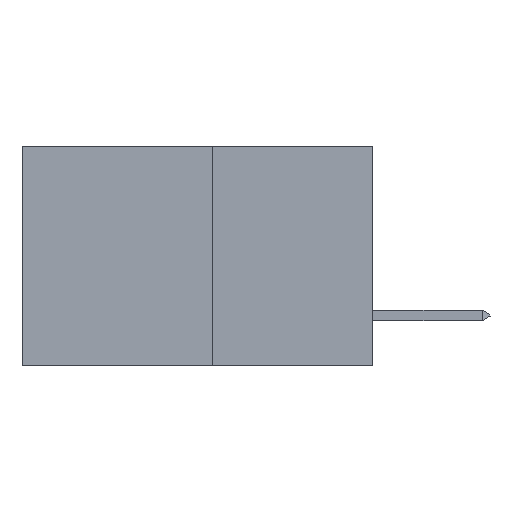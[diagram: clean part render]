
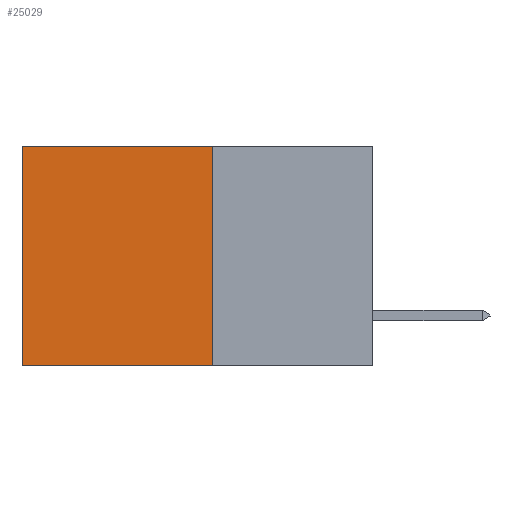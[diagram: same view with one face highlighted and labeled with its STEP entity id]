
A CAD part, left-side view. The second image highlights one B-rep face of the part: STEP entity #25029.
In plain terms, the highlighted planar face has unit normal (-1, 0, 0).
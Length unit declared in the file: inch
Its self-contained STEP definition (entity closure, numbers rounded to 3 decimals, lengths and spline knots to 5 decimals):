
#195 = LINE ( 'NONE', #1239, #15987 ) ;
#360 = LINE ( 'NONE', #1048, #6505 ) ;
#1048 = CARTESIAN_POINT ( 'NONE',  ( 0.277, 0.27, -0.37 ) ) ;
#1239 = CARTESIAN_POINT ( 'NONE',  ( 0.277, 0.27, 0. ) ) ;
#3177 = VERTEX_POINT ( 'NONE', #15548 ) ;
#3860 = CARTESIAN_POINT ( 'NONE',  ( 0.277, 0.27, -0.37 ) ) ;
#5850 = EDGE_LOOP ( 'NONE', ( #11351, #7434, #7591, #14963 ) ) ;
#5979 = DIRECTION ( 'NONE',  ( 0., 0., -1. ) ) ;
#6505 = VECTOR ( 'NONE', #15472, 39.37008 ) ;
#6676 = EDGE_CURVE ( 'NONE', #18423, #24757, #7171, .T. ) ;
#7171 = LINE ( 'NONE', #18884, #12666 ) ;
#7434 = ORIENTED_EDGE ( 'NONE', *, *, #20124, .F. ) ;
#7591 = ORIENTED_EDGE ( 'NONE', *, *, #8019, .F. ) ;
#8019 = EDGE_CURVE ( 'NONE', #16230, #3177, #17352, .T. ) ;
#8940 = AXIS2_PLACEMENT_3D ( 'NONE', #3860, #18240, #5979 ) ;
#11266 = CARTESIAN_POINT ( 'NONE',  ( 0.277, 0.59, -0.37 ) ) ;
#11351 = ORIENTED_EDGE ( 'NONE', *, *, #6676, .T. ) ;
#12666 = VECTOR ( 'NONE', #19053, 39.37008 ) ;
#13149 = CARTESIAN_POINT ( 'NONE',  ( 0.277, 0.27, 0. ) ) ;
#14621 = CARTESIAN_POINT ( 'NONE',  ( 0.277, 0.59, 0. ) ) ;
#14963 = ORIENTED_EDGE ( 'NONE', *, *, #16815, .T. ) ;
#15472 = DIRECTION ( 'NONE',  ( 0., 1., 0. ) ) ;
#15548 = CARTESIAN_POINT ( 'NONE',  ( 0.277, 0.27, -0.37 ) ) ;
#15669 = DIRECTION ( 'NONE',  ( 0., 1., 0. ) ) ;
#15987 = VECTOR ( 'NONE', #15669, 39.37008 ) ;
#16229 = PLANE ( 'NONE',  #8940 ) ;
#16230 = VERTEX_POINT ( 'NONE', #13149 ) ;
#16815 = EDGE_CURVE ( 'NONE', #16230, #18423, #195, .T. ) ;
#16862 = FACE_OUTER_BOUND ( 'NONE', #5850, .T. ) ;
#17352 = LINE ( 'NONE', #24204, #22549 ) ;
#18240 = DIRECTION ( 'NONE',  ( 1., 0., 0. ) ) ;
#18402 = DIRECTION ( 'NONE',  ( 0., 0., -1. ) ) ;
#18423 = VERTEX_POINT ( 'NONE', #14621 ) ;
#18884 = CARTESIAN_POINT ( 'NONE',  ( 0.277, 0.59, -0.37 ) ) ;
#19053 = DIRECTION ( 'NONE',  ( 0., 0., -1. ) ) ;
#20124 = EDGE_CURVE ( 'NONE', #3177, #24757, #360, .T. ) ;
#22549 = VECTOR ( 'NONE', #18402, 39.37008 ) ;
#24204 = CARTESIAN_POINT ( 'NONE',  ( 0.277, 0.27, -0.37 ) ) ;
#24757 = VERTEX_POINT ( 'NONE', #11266 ) ;
#25029 = ADVANCED_FACE ( 'NONE', ( #16862 ), #16229, .F. ) ;
